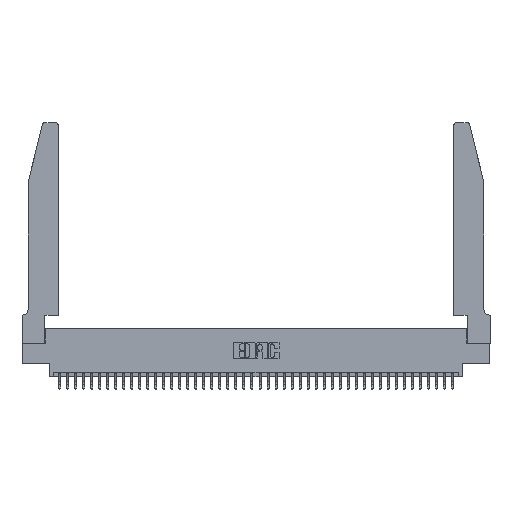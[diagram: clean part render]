
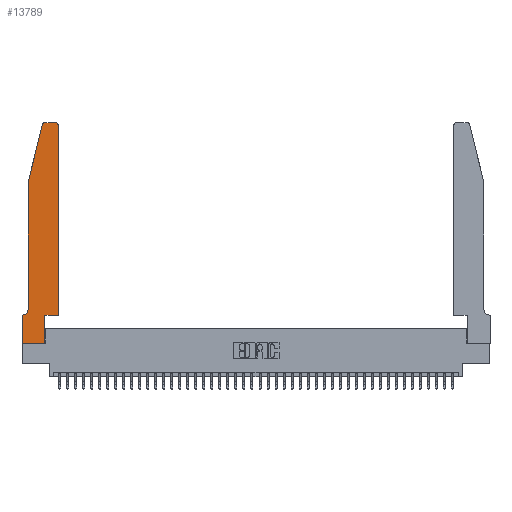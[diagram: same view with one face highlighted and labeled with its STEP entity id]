
A CAD part, top view. The second image highlights one B-rep face of the part: STEP entity #13789.
In plain terms, the highlighted planar face has unit normal (0, 0, 1).
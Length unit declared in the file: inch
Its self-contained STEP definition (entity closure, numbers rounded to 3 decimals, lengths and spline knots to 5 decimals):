
#185 = DIRECTION ( 'NONE',  ( 1., 0., 0. ) ) ;
#187 = CARTESIAN_POINT ( 'NONE',  ( 0.0055, 0.42, 0.37 ) ) ;
#265 = LINE ( 'NONE', #2934, #8208 ) ;
#778 = CARTESIAN_POINT ( 'NONE',  ( 0.4505, 0.35, 0.37 ) ) ;
#1185 = VERTEX_POINT ( 'NONE', #3208 ) ;
#1427 = CARTESIAN_POINT ( 'NONE',  ( 0., 0.35, 0.37 ) ) ;
#1569 = EDGE_CURVE ( 'NONE', #26210, #7971, #17428, .T. ) ;
#1664 = CARTESIAN_POINT ( 'NONE',  ( 0.0755, 2., 0.37 ) ) ;
#2934 = CARTESIAN_POINT ( 'NONE',  ( 0.2605, 2.75, 0.37 ) ) ;
#3143 = CARTESIAN_POINT ( 'NONE',  ( 0.0755, 2., 0.37 ) ) ;
#3208 = CARTESIAN_POINT ( 'NONE',  ( 0.25487, 2.72718, 0.37 ) ) ;
#3578 = DIRECTION ( 'NONE',  ( -1., 0., 0. ) ) ;
#4221 = VECTOR ( 'NONE', #12044, 39.37008 ) ;
#4642 = LINE ( 'NONE', #19827, #30328 ) ;
#5033 = DIRECTION ( 'NONE',  ( 1., 0., 0. ) ) ;
#5079 = ORIENTED_EDGE ( 'NONE', *, *, #33516, .T. ) ;
#5158 = AXIS2_PLACEMENT_3D ( 'NONE', #33974, #14010, #37291 ) ;
#5915 = FACE_OUTER_BOUND ( 'NONE', #31102, .T. ) ;
#5936 = CIRCLE ( 'NONE', #24073, 0.03 ) ;
#6314 = ORIENTED_EDGE ( 'NONE', *, *, #40853, .T. ) ;
#6355 = DIRECTION ( 'NONE',  ( -1., 0., 0. ) ) ;
#6566 = DIRECTION ( 'NONE',  ( 0., -1., 0. ) ) ;
#7916 = VERTEX_POINT ( 'NONE', #36867 ) ;
#7971 = VERTEX_POINT ( 'NONE', #17358 ) ;
#8208 = VECTOR ( 'NONE', #6355, 39.37008 ) ;
#8214 = CARTESIAN_POINT ( 'NONE',  ( 0.2865, 0.35, 0.37 ) ) ;
#8762 = ORIENTED_EDGE ( 'NONE', *, *, #31841, .T. ) ;
#9387 = CIRCLE ( 'NONE', #5158, 0.03 ) ;
#9494 = VERTEX_POINT ( 'NONE', #18287 ) ;
#10192 = VERTEX_POINT ( 'NONE', #15449 ) ;
#11605 = LINE ( 'NONE', #41628, #37132 ) ;
#11711 = CARTESIAN_POINT ( 'NONE',  ( 0., 0.35, 0.37 ) ) ;
#12044 = DIRECTION ( 'NONE',  ( -1., 0., 0. ) ) ;
#13200 = AXIS2_PLACEMENT_3D ( 'NONE', #11711, #25099, #5033 ) ;
#13732 = VECTOR ( 'NONE', #19159, 39.37008 ) ;
#13789 = ADVANCED_FACE ( 'NONE', ( #5915 ), #18416, .T. ) ;
#13802 = LINE ( 'NONE', #1664, #30514 ) ;
#14010 = DIRECTION ( 'NONE',  ( 0., 0., 1. ) ) ;
#14727 = VECTOR ( 'NONE', #36903, 39.37008 ) ;
#15232 = CARTESIAN_POINT ( 'NONE',  ( 0.4205, 2.75, 0.37 ) ) ;
#15449 = CARTESIAN_POINT ( 'NONE',  ( 0.0755, 2., 0.37 ) ) ;
#15889 = VECTOR ( 'NONE', #6566, 39.37008 ) ;
#16686 = ORIENTED_EDGE ( 'NONE', *, *, #18947, .T. ) ;
#16856 = EDGE_CURVE ( 'NONE', #9494, #41740, #22190, .T. ) ;
#16920 = AXIS2_PLACEMENT_3D ( 'NONE', #187, #23668, #3578 ) ;
#17358 = CARTESIAN_POINT ( 'NONE',  ( 0.2865, 0., 0.37 ) ) ;
#17428 = LINE ( 'NONE', #42333, #33076 ) ;
#18287 = CARTESIAN_POINT ( 'NONE',  ( 0.0755, 0.42, 0.37 ) ) ;
#18416 = PLANE ( 'NONE',  #13200 ) ;
#18517 = EDGE_CURVE ( 'NONE', #10192, #9494, #42391, .T. ) ;
#18947 = EDGE_CURVE ( 'NONE', #41740, #26473, #36683, .T. ) ;
#19082 = EDGE_CURVE ( 'NONE', #36128, #21704, #30451, .T. ) ;
#19159 = DIRECTION ( 'NONE',  ( 0., 1., 0. ) ) ;
#19827 = CARTESIAN_POINT ( 'NONE',  ( 0.2865, 0.35, 0.37 ) ) ;
#20348 = DIRECTION ( 'NONE',  ( 0., 0., 1. ) ) ;
#20409 = EDGE_CURVE ( 'NONE', #7971, #24053, #4642, .T. ) ;
#21682 = DIRECTION ( 'NONE',  ( 1., 0., 0. ) ) ;
#21704 = VERTEX_POINT ( 'NONE', #23773 ) ;
#21802 = DIRECTION ( 'NONE',  ( -0.239, -0.971, 0. ) ) ;
#22190 = CIRCLE ( 'NONE', #16920, 0.07 ) ;
#22918 = ORIENTED_EDGE ( 'NONE', *, *, #20409, .T. ) ;
#23386 = ORIENTED_EDGE ( 'NONE', *, *, #38969, .T. ) ;
#23668 = DIRECTION ( 'NONE',  ( 0., 0., -1. ) ) ;
#23773 = CARTESIAN_POINT ( 'NONE',  ( 0.4505, 2.72, 0.37 ) ) ;
#24053 = VERTEX_POINT ( 'NONE', #8214 ) ;
#24073 = AXIS2_PLACEMENT_3D ( 'NONE', #40270, #20348, #185 ) ;
#25099 = DIRECTION ( 'NONE',  ( 0., 0., 1. ) ) ;
#26014 = VERTEX_POINT ( 'NONE', #15232 ) ;
#26150 = ORIENTED_EDGE ( 'NONE', *, *, #28030, .T. ) ;
#26210 = VERTEX_POINT ( 'NONE', #29649 ) ;
#26473 = VERTEX_POINT ( 'NONE', #1427 ) ;
#28030 = EDGE_CURVE ( 'NONE', #26014, #7916, #265, .T. ) ;
#28659 = CARTESIAN_POINT ( 'NONE',  ( 0.0755, 0.35, 0.37 ) ) ;
#29649 = CARTESIAN_POINT ( 'NONE',  ( 0., 0., 0.37 ) ) ;
#30328 = VECTOR ( 'NONE', #43049, 39.37008 ) ;
#30451 = LINE ( 'NONE', #42399, #13732 ) ;
#30514 = VECTOR ( 'NONE', #21802, 39.37008 ) ;
#30522 = EDGE_CURVE ( 'NONE', #1185, #10192, #13802, .T. ) ;
#31102 = EDGE_LOOP ( 'NONE', ( #26150, #5079, #37676, #31860, #40093, #16686, #6314, #32043, #22918, #8762, #40861, #23386 ) ) ;
#31327 = CARTESIAN_POINT ( 'NONE',  ( 0.0055, 0.35, 0.37 ) ) ;
#31841 = EDGE_CURVE ( 'NONE', #24053, #36128, #11605, .T. ) ;
#31860 = ORIENTED_EDGE ( 'NONE', *, *, #18517, .T. ) ;
#32043 = ORIENTED_EDGE ( 'NONE', *, *, #1569, .T. ) ;
#32479 = LINE ( 'NONE', #33574, #14727 ) ;
#32523 = DIRECTION ( 'NONE',  ( 1., 0., 0. ) ) ;
#33076 = VECTOR ( 'NONE', #32523, 39.37008 ) ;
#33516 = EDGE_CURVE ( 'NONE', #7916, #1185, #9387, .T. ) ;
#33574 = CARTESIAN_POINT ( 'NONE',  ( 0., 0., 0.37 ) ) ;
#33974 = CARTESIAN_POINT ( 'NONE',  ( 0.284, 2.72, 0.37 ) ) ;
#36128 = VERTEX_POINT ( 'NONE', #778 ) ;
#36683 = LINE ( 'NONE', #28659, #4221 ) ;
#36867 = CARTESIAN_POINT ( 'NONE',  ( 0.284, 2.75, 0.37 ) ) ;
#36903 = DIRECTION ( 'NONE',  ( 0., -1., 0. ) ) ;
#37132 = VECTOR ( 'NONE', #21682, 39.37008 ) ;
#37291 = DIRECTION ( 'NONE',  ( 1., 0., 0. ) ) ;
#37676 = ORIENTED_EDGE ( 'NONE', *, *, #30522, .T. ) ;
#38969 = EDGE_CURVE ( 'NONE', #21704, #26014, #5936, .T. ) ;
#40093 = ORIENTED_EDGE ( 'NONE', *, *, #16856, .T. ) ;
#40270 = CARTESIAN_POINT ( 'NONE',  ( 0.4205, 2.72, 0.37 ) ) ;
#40853 = EDGE_CURVE ( 'NONE', #26473, #26210, #32479, .T. ) ;
#40861 = ORIENTED_EDGE ( 'NONE', *, *, #19082, .T. ) ;
#41628 = CARTESIAN_POINT ( 'NONE',  ( 0.4505, 0.35, 0.37 ) ) ;
#41740 = VERTEX_POINT ( 'NONE', #31327 ) ;
#42333 = CARTESIAN_POINT ( 'NONE',  ( 0., 0., 0.37 ) ) ;
#42391 = LINE ( 'NONE', #3143, #15889 ) ;
#42399 = CARTESIAN_POINT ( 'NONE',  ( 0.4505, 0.35, 0.37 ) ) ;
#43049 = DIRECTION ( 'NONE',  ( 0., 1., 0. ) ) ;
